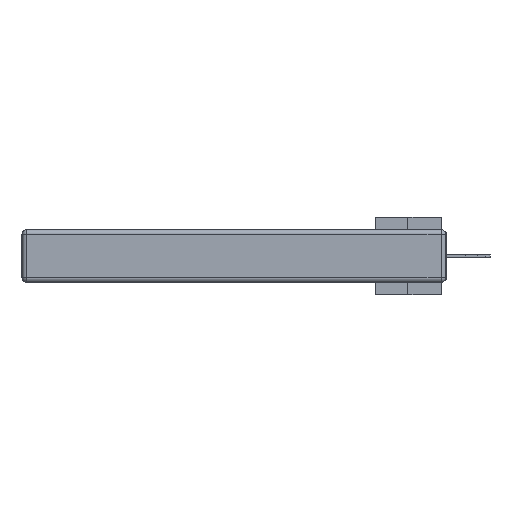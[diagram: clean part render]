
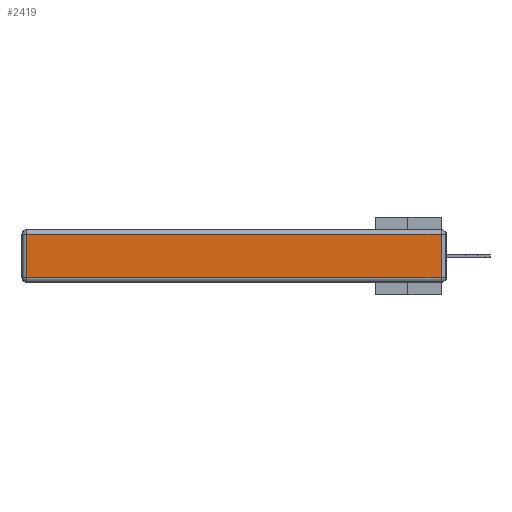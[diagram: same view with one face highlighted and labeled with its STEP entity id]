
A CAD part, left-side view. The second image highlights one B-rep face of the part: STEP entity #2419.
In plain terms, the highlighted planar face has unit normal (-1, 0, 0).
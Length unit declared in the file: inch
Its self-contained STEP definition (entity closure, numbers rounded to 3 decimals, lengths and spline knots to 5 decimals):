
#1409 = DIRECTION ( 'NONE',  ( 0., 0., -1. ) ) ;
#2419 = ADVANCED_FACE ( 'NONE', ( #11267 ), #22994, .T. ) ;
#2586 = EDGE_CURVE ( 'NONE', #23308, #9651, #2791, .T. ) ;
#2791 = LINE ( 'NONE', #28141, #18262 ) ;
#4683 = LINE ( 'NONE', #31991, #35656 ) ;
#5188 = ORIENTED_EDGE ( 'NONE', *, *, #6296, .T. ) ;
#6296 = EDGE_CURVE ( 'NONE', #9651, #23404, #4683, .T. ) ;
#6551 = VECTOR ( 'NONE', #31960, 39.37008 ) ;
#8049 = DIRECTION ( 'NONE',  ( 0., 0., 1. ) ) ;
#8531 = EDGE_LOOP ( 'NONE', ( #5188, #29759, #37762, #34447 ) ) ;
#9651 = VERTEX_POINT ( 'NONE', #16936 ) ;
#10856 = DIRECTION ( 'NONE',  ( 0., 1., 0. ) ) ;
#11267 = FACE_OUTER_BOUND ( 'NONE', #8531, .T. ) ;
#14940 = LINE ( 'NONE', #37920, #6551 ) ;
#15611 = CARTESIAN_POINT ( 'NONE',  ( 0., 2.72, -0.03 ) ) ;
#16936 = CARTESIAN_POINT ( 'NONE',  ( 0., 2.72, -0.313 ) ) ;
#17371 = DIRECTION ( 'NONE',  ( 0., -1., 0. ) ) ;
#18262 = VECTOR ( 'NONE', #1409, 39.37008 ) ;
#19588 = CARTESIAN_POINT ( 'NONE',  ( 0., 2.75, -0.03 ) ) ;
#19681 = EDGE_CURVE ( 'NONE', #36790, #23308, #36901, .T. ) ;
#20889 = VECTOR ( 'NONE', #10856, 39.37008 ) ;
#22615 = EDGE_CURVE ( 'NONE', #23404, #36790, #14940, .T. ) ;
#22994 = PLANE ( 'NONE',  #26607 ) ;
#23308 = VERTEX_POINT ( 'NONE', #15611 ) ;
#23404 = VERTEX_POINT ( 'NONE', #25343 ) ;
#25343 = CARTESIAN_POINT ( 'NONE',  ( 0., 0.03, -0.313 ) ) ;
#25630 = CARTESIAN_POINT ( 'NONE',  ( 0., 0.03, -0.03 ) ) ;
#25769 = DIRECTION ( 'NONE',  ( -1., 0., 0. ) ) ;
#26607 = AXIS2_PLACEMENT_3D ( 'NONE', #28616, #25769, #8049 ) ;
#28141 = CARTESIAN_POINT ( 'NONE',  ( 0., 2.72, -0.343 ) ) ;
#28616 = CARTESIAN_POINT ( 'NONE',  ( 0., 0., -0.343 ) ) ;
#29759 = ORIENTED_EDGE ( 'NONE', *, *, #22615, .T. ) ;
#31960 = DIRECTION ( 'NONE',  ( 0., 0., 1. ) ) ;
#31991 = CARTESIAN_POINT ( 'NONE',  ( 0., 0., -0.313 ) ) ;
#34447 = ORIENTED_EDGE ( 'NONE', *, *, #2586, .T. ) ;
#35656 = VECTOR ( 'NONE', #17371, 39.37008 ) ;
#36790 = VERTEX_POINT ( 'NONE', #25630 ) ;
#36901 = LINE ( 'NONE', #19588, #20889 ) ;
#37762 = ORIENTED_EDGE ( 'NONE', *, *, #19681, .T. ) ;
#37920 = CARTESIAN_POINT ( 'NONE',  ( 0., 0.03, -0.343 ) ) ;
